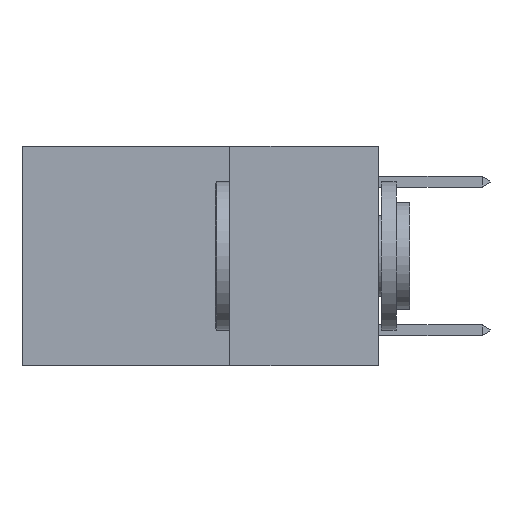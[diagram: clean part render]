
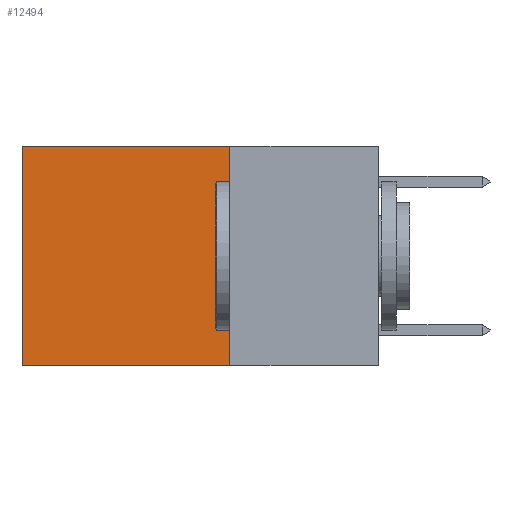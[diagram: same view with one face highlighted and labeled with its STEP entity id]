
A CAD part, left-side view. The second image highlights one B-rep face of the part: STEP entity #12494.
In plain terms, the highlighted planar face has unit normal (-1, 0, 0).
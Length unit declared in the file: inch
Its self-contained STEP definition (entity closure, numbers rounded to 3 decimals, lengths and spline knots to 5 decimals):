
#7 = DIRECTION ( 'NONE',  ( 0., 1., 0. ) ) ;
#149 = LINE ( 'NONE', #1228, #6684 ) ;
#270 = DIRECTION ( 'NONE',  ( 0., 1., 0. ) ) ;
#321 = CARTESIAN_POINT ( 'NONE',  ( 0.2625, 0.25, -0.37 ) ) ;
#515 = DIRECTION ( 'NONE',  ( 1., 0., 0. ) ) ;
#676 = CARTESIAN_POINT ( 'NONE',  ( 0.2625, 0.6, 0. ) ) ;
#719 = DIRECTION ( 'NONE',  ( 0., 0., -1. ) ) ;
#1228 = CARTESIAN_POINT ( 'NONE',  ( 0.2625, 0.25, 0. ) ) ;
#2204 = EDGE_CURVE ( 'NONE', #6653, #5019, #7814, .T. ) ;
#2559 = FACE_OUTER_BOUND ( 'NONE', #7519, .T. ) ;
#3021 = ORIENTED_EDGE ( 'NONE', *, *, #4331, .T. ) ;
#3687 = ORIENTED_EDGE ( 'NONE', *, *, #4762, .T. ) ;
#3820 = VERTEX_POINT ( 'NONE', #676 ) ;
#4030 = VECTOR ( 'NONE', #719, 39.37008 ) ;
#4322 = EDGE_CURVE ( 'NONE', #12213, #6653, #5590, .T. ) ;
#4331 = EDGE_CURVE ( 'NONE', #3820, #5019, #7364, .T. ) ;
#4618 = CARTESIAN_POINT ( 'NONE',  ( 0.2625, 0.25, 0. ) ) ;
#4762 = EDGE_CURVE ( 'NONE', #12213, #3820, #149, .T. ) ;
#4878 = CARTESIAN_POINT ( 'NONE',  ( 0.2625, 0.25, 0. ) ) ;
#5019 = VERTEX_POINT ( 'NONE', #8207 ) ;
#5447 = PLANE ( 'NONE',  #11991 ) ;
#5590 = LINE ( 'NONE', #9415, #4030 ) ;
#6030 = VECTOR ( 'NONE', #7, 39.37008 ) ;
#6413 = CARTESIAN_POINT ( 'NONE',  ( 0.2625, 0.6, 0. ) ) ;
#6653 = VERTEX_POINT ( 'NONE', #321 ) ;
#6684 = VECTOR ( 'NONE', #270, 39.37008 ) ;
#7000 = CARTESIAN_POINT ( 'NONE',  ( 0.2625, 0.25, -0.37 ) ) ;
#7364 = LINE ( 'NONE', #6413, #11318 ) ;
#7519 = EDGE_LOOP ( 'NONE', ( #3021, #8129, #9289, #3687 ) ) ;
#7814 = LINE ( 'NONE', #7000, #6030 ) ;
#8129 = ORIENTED_EDGE ( 'NONE', *, *, #2204, .F. ) ;
#8207 = CARTESIAN_POINT ( 'NONE',  ( 0.2625, 0.6, -0.37 ) ) ;
#8396 = DIRECTION ( 'NONE',  ( 0., 0., -1. ) ) ;
#9289 = ORIENTED_EDGE ( 'NONE', *, *, #4322, .F. ) ;
#9301 = DIRECTION ( 'NONE',  ( 0., 0., -1. ) ) ;
#9415 = CARTESIAN_POINT ( 'NONE',  ( 0.2625, 0.25, 0. ) ) ;
#11318 = VECTOR ( 'NONE', #9301, 39.37008 ) ;
#11991 = AXIS2_PLACEMENT_3D ( 'NONE', #4618, #515, #8396 ) ;
#12213 = VERTEX_POINT ( 'NONE', #4878 ) ;
#12494 = ADVANCED_FACE ( 'NONE', ( #2559 ), #5447, .F. ) ;
